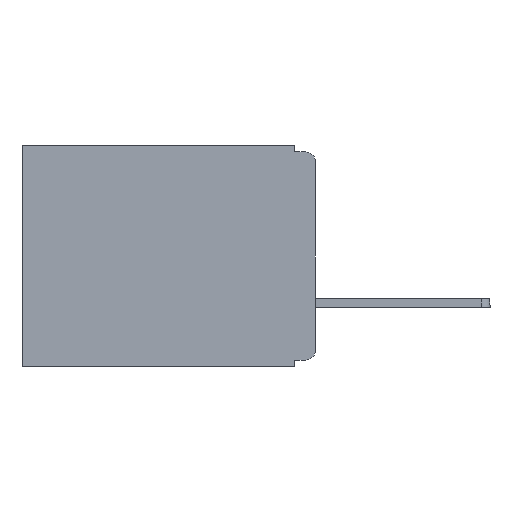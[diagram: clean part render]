
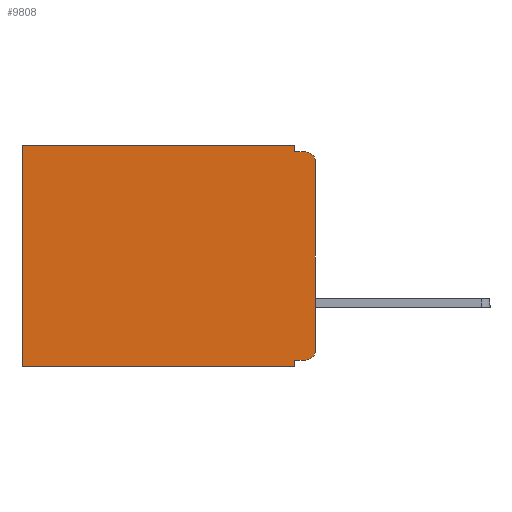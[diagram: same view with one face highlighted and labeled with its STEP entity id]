
A CAD part, left-side view. The second image highlights one B-rep face of the part: STEP entity #9808.
In plain terms, the highlighted planar face has unit normal (-1, 0, 0).
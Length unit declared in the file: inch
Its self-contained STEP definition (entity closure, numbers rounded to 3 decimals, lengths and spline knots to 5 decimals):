
#87 = EDGE_CURVE ( 'NONE', #6962, #30571, #21106, .T. ) ;
#574 = CARTESIAN_POINT ( 'NONE',  ( 0.3, 0., -0.33 ) ) ;
#1682 = DIRECTION ( 'NONE',  ( 0., 1., 0. ) ) ;
#2021 = ORIENTED_EDGE ( 'NONE', *, *, #29139, .F. ) ;
#2314 = VECTOR ( 'NONE', #15257, 39.37008 ) ;
#2348 = VERTEX_POINT ( 'NONE', #12234 ) ;
#2714 = LINE ( 'NONE', #9081, #15689 ) ;
#2888 = ORIENTED_EDGE ( 'NONE', *, *, #87, .F. ) ;
#3926 = CARTESIAN_POINT ( 'NONE',  ( 0.3, 0.031, -0.33 ) ) ;
#4072 = CARTESIAN_POINT ( 'NONE',  ( 0.3, 0.015, -0.025 ) ) ;
#5240 = DIRECTION ( 'NONE',  ( 0., 1., 0. ) ) ;
#5374 = EDGE_CURVE ( 'NONE', #12588, #25438, #23702, .T. ) ;
#5460 = CARTESIAN_POINT ( 'NONE',  ( 0.3, 0.437, -0.33 ) ) ;
#5487 = PLANE ( 'NONE',  #25424 ) ;
#5614 = CARTESIAN_POINT ( 'NONE',  ( 0.3, 0., -0.025 ) ) ;
#5842 = VECTOR ( 'NONE', #16272, 39.37008 ) ;
#5994 = ORIENTED_EDGE ( 'NONE', *, *, #16573, .F. ) ;
#6542 = DIRECTION ( 'NONE',  ( 0., 0., -1. ) ) ;
#6962 = VERTEX_POINT ( 'NONE', #5614 ) ;
#7059 = VERTEX_POINT ( 'NONE', #18192 ) ;
#7092 = CARTESIAN_POINT ( 'NONE',  ( 0.3, 0., -0.305 ) ) ;
#7931 = DIRECTION ( 'NONE',  ( 0., 0., -1. ) ) ;
#7970 = CARTESIAN_POINT ( 'NONE',  ( 0.3, 0.031, 0. ) ) ;
#7974 = DIRECTION ( 'NONE',  ( 1., 0., 0. ) ) ;
#8029 = VERTEX_POINT ( 'NONE', #7970 ) ;
#8418 = VERTEX_POINT ( 'NONE', #19115 ) ;
#9081 = CARTESIAN_POINT ( 'NONE',  ( 0.3, 0., 0. ) ) ;
#9614 = LINE ( 'NONE', #27240, #2314 ) ;
#9808 = ADVANCED_FACE ( 'NONE', ( #26270 ), #5487, .F. ) ;
#10088 = AXIS2_PLACEMENT_3D ( 'NONE', #4072, #21095, #6542 ) ;
#10185 = CARTESIAN_POINT ( 'NONE',  ( 0.3, 0., -0.33 ) ) ;
#10212 = DIRECTION ( 'NONE',  ( 0., 0., -1. ) ) ;
#10296 = LINE ( 'NONE', #3926, #28096 ) ;
#11598 = VECTOR ( 'NONE', #5240, 39.37008 ) ;
#11929 = VECTOR ( 'NONE', #7931, 39.37008 ) ;
#12234 = CARTESIAN_POINT ( 'NONE',  ( 0.3, 0.437, 0. ) ) ;
#12585 = DIRECTION ( 'NONE',  ( -1., 0., 0. ) ) ;
#12588 = VERTEX_POINT ( 'NONE', #12749 ) ;
#12647 = ORIENTED_EDGE ( 'NONE', *, *, #15409, .T. ) ;
#12749 = CARTESIAN_POINT ( 'NONE',  ( 0.3, 0.031, -0.01 ) ) ;
#13384 = CARTESIAN_POINT ( 'NONE',  ( 0.3, 0., -0.33 ) ) ;
#13901 = CIRCLE ( 'NONE', #29035, 0.015 ) ;
#14532 = CARTESIAN_POINT ( 'NONE',  ( 0.3, 0.437, -0.33 ) ) ;
#14644 = VECTOR ( 'NONE', #10212, 39.37008 ) ;
#15257 = DIRECTION ( 'NONE',  ( 0., 0., -1. ) ) ;
#15409 = EDGE_CURVE ( 'NONE', #8029, #2348, #2714, .T. ) ;
#15689 = VECTOR ( 'NONE', #1682, 39.37008 ) ;
#16056 = ORIENTED_EDGE ( 'NONE', *, *, #22407, .F. ) ;
#16272 = DIRECTION ( 'NONE',  ( 0., -1., 0. ) ) ;
#16573 = EDGE_CURVE ( 'NONE', #7059, #22427, #10296, .T. ) ;
#18077 = LINE ( 'NONE', #19828, #11598 ) ;
#18192 = CARTESIAN_POINT ( 'NONE',  ( 0.3, 0.031, -0.32 ) ) ;
#18393 = LINE ( 'NONE', #5460, #11929 ) ;
#19115 = CARTESIAN_POINT ( 'NONE',  ( 0.3, 0.015, -0.32 ) ) ;
#19828 = CARTESIAN_POINT ( 'NONE',  ( 0.3, 0., -0.32 ) ) ;
#20081 = EDGE_CURVE ( 'NONE', #8418, #30571, #13901, .T. ) ;
#20599 = CIRCLE ( 'NONE', #10088, 0.015 ) ;
#20659 = ORIENTED_EDGE ( 'NONE', *, *, #30765, .T. ) ;
#20921 = ORIENTED_EDGE ( 'NONE', *, *, #20081, .T. ) ;
#21095 = DIRECTION ( 'NONE',  ( -1., 0., 0. ) ) ;
#21106 = LINE ( 'NONE', #10185, #14644 ) ;
#21888 = VECTOR ( 'NONE', #30485, 39.37008 ) ;
#22239 = VERTEX_POINT ( 'NONE', #14532 ) ;
#22407 = EDGE_CURVE ( 'NONE', #8029, #12588, #9614, .T. ) ;
#22427 = VERTEX_POINT ( 'NONE', #27449 ) ;
#22613 = EDGE_CURVE ( 'NONE', #6962, #25438, #20599, .T. ) ;
#22888 = ORIENTED_EDGE ( 'NONE', *, *, #27218, .F. ) ;
#23702 = LINE ( 'NONE', #30688, #5842 ) ;
#24948 = DIRECTION ( 'NONE',  ( 0., 0., -1. ) ) ;
#25424 = AXIS2_PLACEMENT_3D ( 'NONE', #574, #7974, #24948 ) ;
#25438 = VERTEX_POINT ( 'NONE', #31457 ) ;
#25713 = DIRECTION ( 'NONE',  ( 0., 0., -1. ) ) ;
#26270 = FACE_OUTER_BOUND ( 'NONE', #26740, .T. ) ;
#26740 = EDGE_LOOP ( 'NONE', ( #2888, #30326, #29931, #16056, #12647, #20659, #2021, #5994, #22888, #20921 ) ) ;
#27082 = CARTESIAN_POINT ( 'NONE',  ( 0.3, 0.015, -0.305 ) ) ;
#27218 = EDGE_CURVE ( 'NONE', #8418, #7059, #18077, .T. ) ;
#27240 = CARTESIAN_POINT ( 'NONE',  ( 0.3, 0.031, 0. ) ) ;
#27449 = CARTESIAN_POINT ( 'NONE',  ( 0.3, 0.031, -0.33 ) ) ;
#28096 = VECTOR ( 'NONE', #25713, 39.37008 ) ;
#28285 = LINE ( 'NONE', #13384, #21888 ) ;
#29035 = AXIS2_PLACEMENT_3D ( 'NONE', #27082, #12585, #29475 ) ;
#29139 = EDGE_CURVE ( 'NONE', #22427, #22239, #28285, .T. ) ;
#29475 = DIRECTION ( 'NONE',  ( 0., 0., -1. ) ) ;
#29931 = ORIENTED_EDGE ( 'NONE', *, *, #5374, .F. ) ;
#30326 = ORIENTED_EDGE ( 'NONE', *, *, #22613, .T. ) ;
#30485 = DIRECTION ( 'NONE',  ( 0., 1., 0. ) ) ;
#30571 = VERTEX_POINT ( 'NONE', #7092 ) ;
#30688 = CARTESIAN_POINT ( 'NONE',  ( 0.3, 0., -0.01 ) ) ;
#30765 = EDGE_CURVE ( 'NONE', #2348, #22239, #18393, .T. ) ;
#31457 = CARTESIAN_POINT ( 'NONE',  ( 0.3, 0.015, -0.01 ) ) ;
